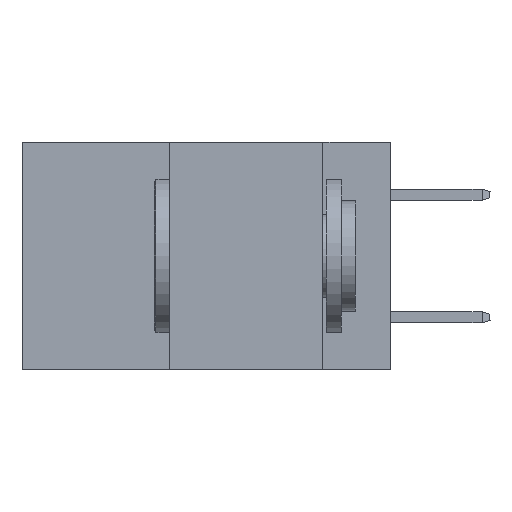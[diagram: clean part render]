
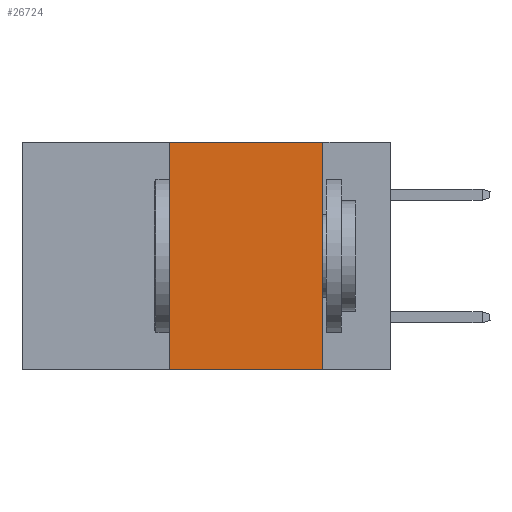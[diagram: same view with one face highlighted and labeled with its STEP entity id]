
A CAD part, left-side view. The second image highlights one B-rep face of the part: STEP entity #26724.
In plain terms, the highlighted planar face has unit normal (-1, 0, 0).
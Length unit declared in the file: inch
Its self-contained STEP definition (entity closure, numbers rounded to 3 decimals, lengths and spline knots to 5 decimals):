
#1298 = CARTESIAN_POINT ( 'NONE',  ( 0., 0.36, -0.37 ) ) ;
#1906 = LINE ( 'NONE', #20940, #32507 ) ;
#2231 = CARTESIAN_POINT ( 'NONE',  ( 0., 0.11, 0. ) ) ;
#3075 = DIRECTION ( 'NONE',  ( 0., 0., 1. ) ) ;
#4239 = VECTOR ( 'NONE', #22777, 39.37008 ) ;
#4387 = DIRECTION ( 'NONE',  ( 1., 0., 0. ) ) ;
#4721 = LINE ( 'NONE', #8510, #4239 ) ;
#4778 = VERTEX_POINT ( 'NONE', #1298 ) ;
#8218 = CARTESIAN_POINT ( 'NONE',  ( 0., 0.11, -0.37 ) ) ;
#8510 = CARTESIAN_POINT ( 'NONE',  ( 0., 0.6, -0.37 ) ) ;
#9604 = LINE ( 'NONE', #31770, #18346 ) ;
#10507 = VERTEX_POINT ( 'NONE', #8218 ) ;
#12556 = EDGE_CURVE ( 'NONE', #4778, #19968, #1906, .T. ) ;
#14494 = VERTEX_POINT ( 'NONE', #2231 ) ;
#17004 = EDGE_CURVE ( 'NONE', #19968, #14494, #9604, .T. ) ;
#17403 = ORIENTED_EDGE ( 'NONE', *, *, #22673, .F. ) ;
#18304 = FACE_OUTER_BOUND ( 'NONE', #28780, .T. ) ;
#18346 = VECTOR ( 'NONE', #25644, 39.37008 ) ;
#19968 = VERTEX_POINT ( 'NONE', #34952 ) ;
#20877 = LINE ( 'NONE', #31520, #29711 ) ;
#20940 = CARTESIAN_POINT ( 'NONE',  ( 0., 0.36, 0. ) ) ;
#22673 = EDGE_CURVE ( 'NONE', #14494, #10507, #20877, .T. ) ;
#22777 = DIRECTION ( 'NONE',  ( 0., -1., 0. ) ) ;
#25644 = DIRECTION ( 'NONE',  ( 0., -1., 0. ) ) ;
#26724 = ADVANCED_FACE ( 'NONE', ( #18304 ), #36653, .F. ) ;
#27132 = ORIENTED_EDGE ( 'NONE', *, *, #12556, .F. ) ;
#27699 = CARTESIAN_POINT ( 'NONE',  ( 0., 0.6, 0. ) ) ;
#28366 = EDGE_CURVE ( 'NONE', #4778, #10507, #4721, .T. ) ;
#28780 = EDGE_LOOP ( 'NONE', ( #17403, #31779, #27132, #37404 ) ) ;
#29711 = VECTOR ( 'NONE', #31795, 39.37008 ) ;
#30447 = AXIS2_PLACEMENT_3D ( 'NONE', #27699, #4387, #33678 ) ;
#31520 = CARTESIAN_POINT ( 'NONE',  ( 0., 0.11, 0. ) ) ;
#31770 = CARTESIAN_POINT ( 'NONE',  ( 0., 0.6, 0. ) ) ;
#31779 = ORIENTED_EDGE ( 'NONE', *, *, #17004, .F. ) ;
#31795 = DIRECTION ( 'NONE',  ( 0., 0., -1. ) ) ;
#32507 = VECTOR ( 'NONE', #3075, 39.37008 ) ;
#33678 = DIRECTION ( 'NONE',  ( 0., 0., -1. ) ) ;
#34952 = CARTESIAN_POINT ( 'NONE',  ( 0., 0.36, 0. ) ) ;
#36653 = PLANE ( 'NONE',  #30447 ) ;
#37404 = ORIENTED_EDGE ( 'NONE', *, *, #28366, .T. ) ;
